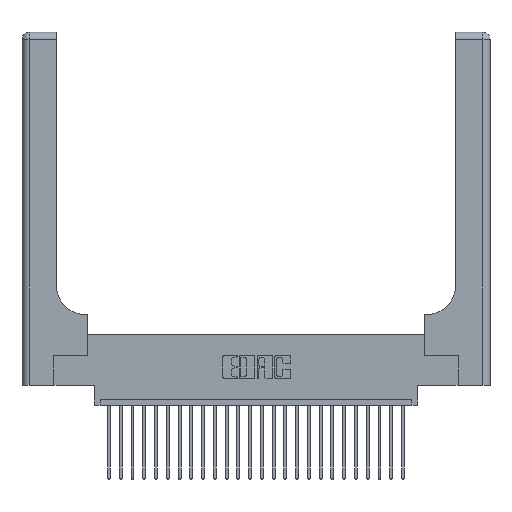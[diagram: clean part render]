
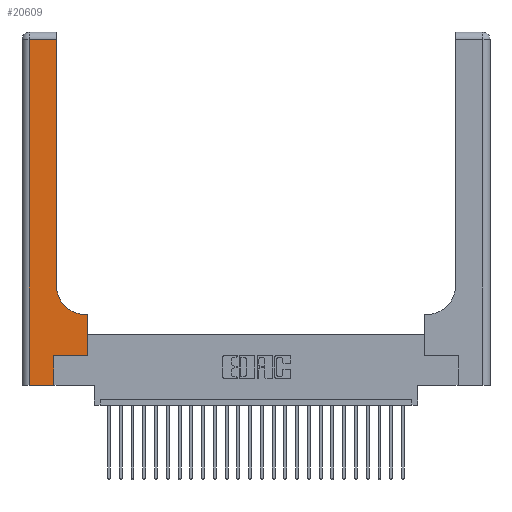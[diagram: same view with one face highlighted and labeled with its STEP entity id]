
A CAD part, top view. The second image highlights one B-rep face of the part: STEP entity #20609.
In plain terms, the highlighted planar face has unit normal (0, 0, 1).
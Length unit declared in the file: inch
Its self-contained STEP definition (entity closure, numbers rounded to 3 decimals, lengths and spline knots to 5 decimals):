
#263 = CARTESIAN_POINT ( 'NONE',  ( 0.2915, 0.6, 0.37 ) ) ;
#602 = VECTOR ( 'NONE', #20536, 39.37008 ) ;
#641 = CARTESIAN_POINT ( 'NONE',  ( 0.06, 3., 0.37 ) ) ;
#792 = ORIENTED_EDGE ( 'NONE', *, *, #17108, .T. ) ;
#950 = LINE ( 'NONE', #641, #4240 ) ;
#1312 = DIRECTION ( 'NONE',  ( 0., 1., 0. ) ) ;
#2028 = ORIENTED_EDGE ( 'NONE', *, *, #6039, .T. ) ;
#3766 = LINE ( 'NONE', #12890, #6390 ) ;
#4240 = VECTOR ( 'NONE', #11879, 39.37008 ) ;
#4295 = LINE ( 'NONE', #14641, #14761 ) ;
#4351 = VERTEX_POINT ( 'NONE', #11460 ) ;
#4388 = VECTOR ( 'NONE', #5614, 39.37008 ) ;
#5106 = DIRECTION ( 'NONE',  ( -1., 0., 0. ) ) ;
#5385 = DIRECTION ( 'NONE',  ( 0., 0., -1. ) ) ;
#5614 = DIRECTION ( 'NONE',  ( 0., 1., 0. ) ) ;
#5804 = ORIENTED_EDGE ( 'NONE', *, *, #12700, .T. ) ;
#5965 = VERTEX_POINT ( 'NONE', #20095 ) ;
#6039 = EDGE_CURVE ( 'NONE', #11323, #5965, #4295, .T. ) ;
#6390 = VECTOR ( 'NONE', #1312, 39.37008 ) ;
#6762 = PLANE ( 'NONE',  #10799 ) ;
#6831 = DIRECTION ( 'NONE',  ( 1., 0., 0. ) ) ;
#6877 = CARTESIAN_POINT ( 'NONE',  ( 0.5585, 0.6, 0.37 ) ) ;
#6942 = ORIENTED_EDGE ( 'NONE', *, *, #12198, .T. ) ;
#7146 = LINE ( 'NONE', #18314, #602 ) ;
#7656 = VERTEX_POINT ( 'NONE', #10979 ) ;
#7941 = DIRECTION ( 'NONE',  ( 0., 0., -1. ) ) ;
#8437 = CARTESIAN_POINT ( 'NONE',  ( 0.06, 0., 0.37 ) ) ;
#8867 = CARTESIAN_POINT ( 'NONE',  ( 0., 3., 0.37 ) ) ;
#9500 = VERTEX_POINT ( 'NONE', #6877 ) ;
#10029 = DIRECTION ( 'NONE',  ( 1., 0., 0. ) ) ;
#10456 = CARTESIAN_POINT ( 'NONE',  ( 0.269, 0.25, 0.37 ) ) ;
#10799 = AXIS2_PLACEMENT_3D ( 'NONE', #8867, #5385, #5106 ) ;
#10979 = CARTESIAN_POINT ( 'NONE',  ( 0.2915, 0.85, 0.37 ) ) ;
#11160 = ORIENTED_EDGE ( 'NONE', *, *, #12407, .T. ) ;
#11323 = VERTEX_POINT ( 'NONE', #19363 ) ;
#11460 = CARTESIAN_POINT ( 'NONE',  ( 0.5585, 0.25, 0.37 ) ) ;
#11879 = DIRECTION ( 'NONE',  ( 0., -1., 0. ) ) ;
#12198 = EDGE_CURVE ( 'NONE', #16676, #21410, #13103, .T. ) ;
#12407 = EDGE_CURVE ( 'NONE', #5965, #16676, #950, .T. ) ;
#12700 = EDGE_CURVE ( 'NONE', #7656, #11323, #7146, .T. ) ;
#12890 = CARTESIAN_POINT ( 'NONE',  ( 0.5585, 0.25, 0.37 ) ) ;
#13103 = LINE ( 'NONE', #25817, #26132 ) ;
#13128 = ORIENTED_EDGE ( 'NONE', *, *, #14863, .T. ) ;
#13505 = ORIENTED_EDGE ( 'NONE', *, *, #20348, .T. ) ;
#14247 = CARTESIAN_POINT ( 'NONE',  ( 0.5415, 0.85, 0.37 ) ) ;
#14405 = CARTESIAN_POINT ( 'NONE',  ( 0.5415, 0.6, 0.37 ) ) ;
#14641 = CARTESIAN_POINT ( 'NONE',  ( 0., 2.94, 0.37 ) ) ;
#14724 = EDGE_LOOP ( 'NONE', ( #5804, #2028, #11160, #6942, #16775, #792, #13128, #13505, #24536 ) ) ;
#14761 = VECTOR ( 'NONE', #23065, 39.37008 ) ;
#14804 = LINE ( 'NONE', #10456, #25537 ) ;
#14863 = EDGE_CURVE ( 'NONE', #4351, #9500, #3766, .T. ) ;
#15531 = EDGE_CURVE ( 'NONE', #24847, #7656, #16507, .T. ) ;
#15621 = LINE ( 'NONE', #263, #22834 ) ;
#15856 = EDGE_CURVE ( 'NONE', #21410, #25486, #22062, .T. ) ;
#16507 = CIRCLE ( 'NONE', #22245, 0.25 ) ;
#16676 = VERTEX_POINT ( 'NONE', #8437 ) ;
#16775 = ORIENTED_EDGE ( 'NONE', *, *, #15856, .T. ) ;
#17108 = EDGE_CURVE ( 'NONE', #25486, #4351, #14804, .T. ) ;
#18314 = CARTESIAN_POINT ( 'NONE',  ( 0.2915, 3., 0.37 ) ) ;
#18860 = DIRECTION ( 'NONE',  ( 1., 0., 0. ) ) ;
#19363 = CARTESIAN_POINT ( 'NONE',  ( 0.2915, 2.94, 0.37 ) ) ;
#20095 = CARTESIAN_POINT ( 'NONE',  ( 0.06, 2.94, 0.37 ) ) ;
#20161 = CARTESIAN_POINT ( 'NONE',  ( 0.269, 0., 0.37 ) ) ;
#20346 = CARTESIAN_POINT ( 'NONE',  ( 0.269, 0.25, 0.37 ) ) ;
#20348 = EDGE_CURVE ( 'NONE', #9500, #24847, #15621, .T. ) ;
#20536 = DIRECTION ( 'NONE',  ( 0., 1., 0. ) ) ;
#20609 = ADVANCED_FACE ( 'NONE', ( #21205 ), #6762, .F. ) ;
#21205 = FACE_OUTER_BOUND ( 'NONE', #14724, .T. ) ;
#21410 = VERTEX_POINT ( 'NONE', #20161 ) ;
#22062 = LINE ( 'NONE', #24278, #4388 ) ;
#22245 = AXIS2_PLACEMENT_3D ( 'NONE', #14247, #7941, #10029 ) ;
#22834 = VECTOR ( 'NONE', #25373, 39.37008 ) ;
#23065 = DIRECTION ( 'NONE',  ( -1., 0., 0. ) ) ;
#24278 = CARTESIAN_POINT ( 'NONE',  ( 0.269, 0., 0.37 ) ) ;
#24536 = ORIENTED_EDGE ( 'NONE', *, *, #15531, .T. ) ;
#24847 = VERTEX_POINT ( 'NONE', #14405 ) ;
#25373 = DIRECTION ( 'NONE',  ( -1., 0., 0. ) ) ;
#25486 = VERTEX_POINT ( 'NONE', #20346 ) ;
#25537 = VECTOR ( 'NONE', #18860, 39.37008 ) ;
#25817 = CARTESIAN_POINT ( 'NONE',  ( 0., 0., 0.37 ) ) ;
#26132 = VECTOR ( 'NONE', #6831, 39.37008 ) ;
